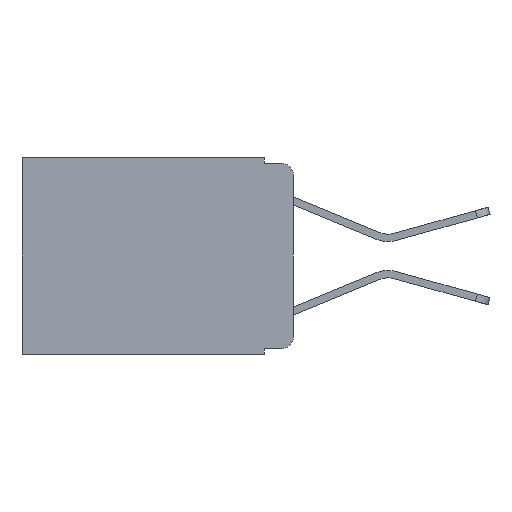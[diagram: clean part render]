
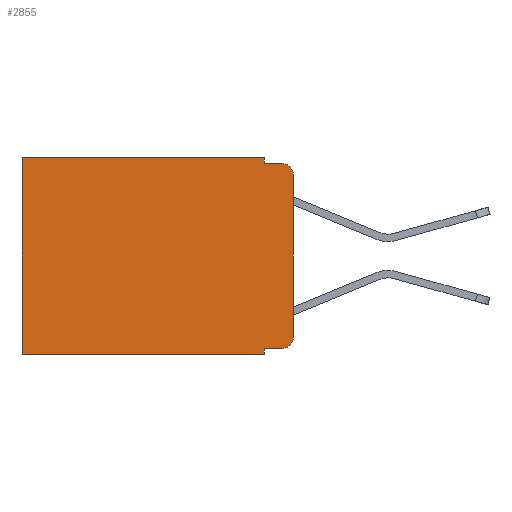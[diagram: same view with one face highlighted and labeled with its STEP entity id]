
A CAD part, left-side view. The second image highlights one B-rep face of the part: STEP entity #2855.
In plain terms, the highlighted planar face has unit normal (-1, 0, 0).
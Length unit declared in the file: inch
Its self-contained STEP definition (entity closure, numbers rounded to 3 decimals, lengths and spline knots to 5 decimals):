
#1109 = ORIENTED_EDGE ( 'NONE', *, *, #5697, .F. ) ;
#1198 = CIRCLE ( 'NONE', #15100, 0.02 ) ;
#1340 = EDGE_CURVE ( 'NONE', #13107, #9250, #2225, .T. ) ;
#1551 = VERTEX_POINT ( 'NONE', #8477 ) ;
#1581 = VERTEX_POINT ( 'NONE', #18706 ) ;
#1852 = ORIENTED_EDGE ( 'NONE', *, *, #2551, .F. ) ;
#2096 = VECTOR ( 'NONE', #3481, 39.37008 ) ;
#2225 = LINE ( 'NONE', #18917, #5893 ) ;
#2357 = ORIENTED_EDGE ( 'NONE', *, *, #12505, .T. ) ;
#2378 = CARTESIAN_POINT ( 'NONE',  ( 0.298, 0.473, -0.343 ) ) ;
#2528 = CARTESIAN_POINT ( 'NONE',  ( 0.298, 0., 0. ) ) ;
#2551 = EDGE_CURVE ( 'NONE', #15462, #1551, #9626, .T. ) ;
#2713 = DIRECTION ( 'NONE',  ( -1., 0., 0. ) ) ;
#2842 = ORIENTED_EDGE ( 'NONE', *, *, #15152, .F. ) ;
#2855 = ADVANCED_FACE ( 'NONE', ( #7373 ), #9140, .F. ) ;
#3340 = ORIENTED_EDGE ( 'NONE', *, *, #18145, .T. ) ;
#3427 = LINE ( 'NONE', #14415, #7110 ) ;
#3481 = DIRECTION ( 'NONE',  ( 0., 0., -1. ) ) ;
#3570 = CARTESIAN_POINT ( 'NONE',  ( 0.298, 0.02, -0.03 ) ) ;
#4135 = CARTESIAN_POINT ( 'NONE',  ( 0.298, 0., -0.313 ) ) ;
#4685 = CARTESIAN_POINT ( 'NONE',  ( 0.298, 0.051, 0. ) ) ;
#4859 = VECTOR ( 'NONE', #11895, 39.37008 ) ;
#4895 = CARTESIAN_POINT ( 'NONE',  ( 0.298, 0.051, -0.01 ) ) ;
#4995 = CARTESIAN_POINT ( 'NONE',  ( 0.298, 0.473, 0. ) ) ;
#5152 = DIRECTION ( 'NONE',  ( 0., 0., -1. ) ) ;
#5422 = CIRCLE ( 'NONE', #6941, 0.02 ) ;
#5546 = ORIENTED_EDGE ( 'NONE', *, *, #12311, .T. ) ;
#5644 = LINE ( 'NONE', #7793, #13840 ) ;
#5697 = EDGE_CURVE ( 'NONE', #1551, #18315, #12597, .T. ) ;
#5893 = VECTOR ( 'NONE', #18959, 39.37008 ) ;
#6941 = AXIS2_PLACEMENT_3D ( 'NONE', #3570, #14357, #5152 ) ;
#7105 = DIRECTION ( 'NONE',  ( 0., 1., 0. ) ) ;
#7110 = VECTOR ( 'NONE', #7105, 39.37008 ) ;
#7373 = FACE_OUTER_BOUND ( 'NONE', #8359, .T. ) ;
#7517 = ORIENTED_EDGE ( 'NONE', *, *, #16500, .T. ) ;
#7793 = CARTESIAN_POINT ( 'NONE',  ( 0.298, 0.051, -0.333 ) ) ;
#8359 = EDGE_LOOP ( 'NONE', ( #16966, #5546, #1109, #1852, #7517, #3340, #2842, #15111, #2357, #10732 ) ) ;
#8477 = CARTESIAN_POINT ( 'NONE',  ( 0.298, 0.051, -0.01 ) ) ;
#8482 = LINE ( 'NONE', #9025, #19893 ) ;
#8525 = CARTESIAN_POINT ( 'NONE',  ( 0.298, 0.02, -0.01 ) ) ;
#8829 = VERTEX_POINT ( 'NONE', #12483 ) ;
#9025 = CARTESIAN_POINT ( 'NONE',  ( 0.298, 0.051, 0. ) ) ;
#9120 = CARTESIAN_POINT ( 'NONE',  ( 0.298, 0.051, -0.343 ) ) ;
#9128 = VECTOR ( 'NONE', #19038, 39.37008 ) ;
#9140 = PLANE ( 'NONE',  #11420 ) ;
#9187 = CARTESIAN_POINT ( 'NONE',  ( 0.298, 0., 0. ) ) ;
#9188 = CARTESIAN_POINT ( 'NONE',  ( 0.298, 0.051, 0. ) ) ;
#9250 = VERTEX_POINT ( 'NONE', #4135 ) ;
#9567 = VERTEX_POINT ( 'NONE', #9120 ) ;
#9626 = LINE ( 'NONE', #9188, #9128 ) ;
#9930 = VERTEX_POINT ( 'NONE', #12916 ) ;
#10732 = ORIENTED_EDGE ( 'NONE', *, *, #12367, .T. ) ;
#11420 = AXIS2_PLACEMENT_3D ( 'NONE', #9187, #18708, #19746 ) ;
#11895 = DIRECTION ( 'NONE',  ( 0., 1., 0. ) ) ;
#12082 = CARTESIAN_POINT ( 'NONE',  ( 0.298, 0.02, -0.313 ) ) ;
#12311 = EDGE_CURVE ( 'NONE', #13107, #18315, #5422, .T. ) ;
#12367 = EDGE_CURVE ( 'NONE', #1581, #9250, #1198, .T. ) ;
#12483 = CARTESIAN_POINT ( 'NONE',  ( 0.298, 0.051, -0.333 ) ) ;
#12505 = EDGE_CURVE ( 'NONE', #8829, #1581, #5644, .T. ) ;
#12597 = LINE ( 'NONE', #4895, #16003 ) ;
#12916 = CARTESIAN_POINT ( 'NONE',  ( 0.298, 0.473, 0. ) ) ;
#13107 = VERTEX_POINT ( 'NONE', #18281 ) ;
#13558 = DIRECTION ( 'NONE',  ( 0., 0., -1. ) ) ;
#13582 = LINE ( 'NONE', #2528, #4859 ) ;
#13840 = VECTOR ( 'NONE', #18306, 39.37008 ) ;
#13952 = VERTEX_POINT ( 'NONE', #2378 ) ;
#14178 = DIRECTION ( 'NONE',  ( 0., -1., 0. ) ) ;
#14357 = DIRECTION ( 'NONE',  ( -1., 0., 0. ) ) ;
#14415 = CARTESIAN_POINT ( 'NONE',  ( 0.298, 0., -0.343 ) ) ;
#14418 = LINE ( 'NONE', #4995, #2096 ) ;
#15100 = AXIS2_PLACEMENT_3D ( 'NONE', #12082, #2713, #13558 ) ;
#15111 = ORIENTED_EDGE ( 'NONE', *, *, #19146, .F. ) ;
#15152 = EDGE_CURVE ( 'NONE', #9567, #13952, #3427, .T. ) ;
#15462 = VERTEX_POINT ( 'NONE', #4685 ) ;
#16003 = VECTOR ( 'NONE', #14178, 39.37008 ) ;
#16500 = EDGE_CURVE ( 'NONE', #15462, #9930, #13582, .T. ) ;
#16966 = ORIENTED_EDGE ( 'NONE', *, *, #1340, .F. ) ;
#18085 = DIRECTION ( 'NONE',  ( 0., 0., -1. ) ) ;
#18145 = EDGE_CURVE ( 'NONE', #9930, #13952, #14418, .T. ) ;
#18281 = CARTESIAN_POINT ( 'NONE',  ( 0.298, 0., -0.03 ) ) ;
#18306 = DIRECTION ( 'NONE',  ( 0., -1., 0. ) ) ;
#18315 = VERTEX_POINT ( 'NONE', #8525 ) ;
#18706 = CARTESIAN_POINT ( 'NONE',  ( 0.298, 0.02, -0.333 ) ) ;
#18708 = DIRECTION ( 'NONE',  ( 1., 0., 0. ) ) ;
#18917 = CARTESIAN_POINT ( 'NONE',  ( 0.298, 0., 0. ) ) ;
#18959 = DIRECTION ( 'NONE',  ( 0., 0., -1. ) ) ;
#19038 = DIRECTION ( 'NONE',  ( 0., 0., -1. ) ) ;
#19146 = EDGE_CURVE ( 'NONE', #8829, #9567, #8482, .T. ) ;
#19746 = DIRECTION ( 'NONE',  ( 0., 0., -1. ) ) ;
#19893 = VECTOR ( 'NONE', #18085, 39.37008 ) ;
